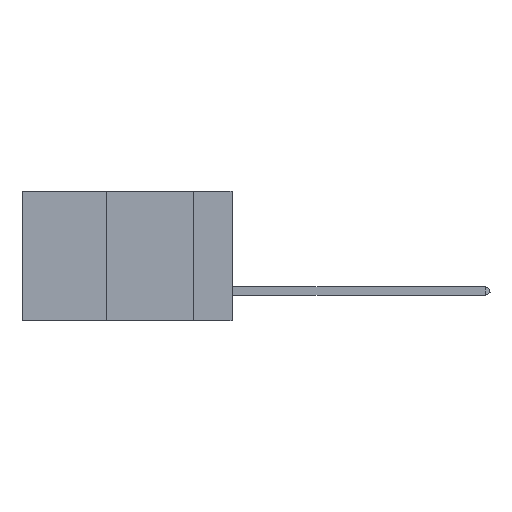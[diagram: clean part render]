
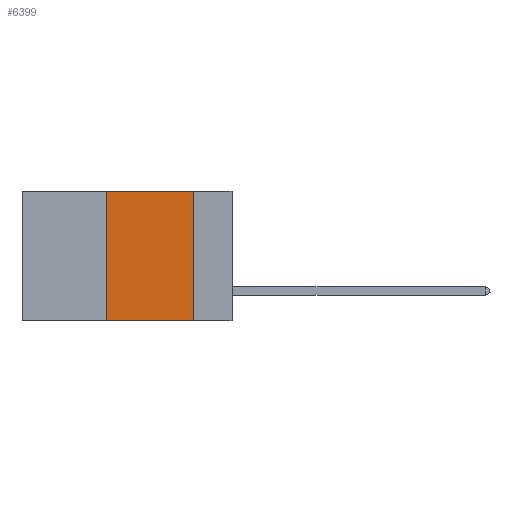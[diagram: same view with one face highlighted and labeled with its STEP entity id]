
A CAD part, left-side view. The second image highlights one B-rep face of the part: STEP entity #6399.
In plain terms, the highlighted planar face has unit normal (-1, 0, 0).
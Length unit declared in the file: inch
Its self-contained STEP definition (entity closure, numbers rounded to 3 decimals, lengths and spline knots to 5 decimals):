
#733 = ORIENTED_EDGE ( 'NONE', *, *, #5323, .T. ) ;
#735 = VECTOR ( 'NONE', #2194, 39.37008 ) ;
#1109 = ORIENTED_EDGE ( 'NONE', *, *, #1247, .F. ) ;
#1247 = EDGE_CURVE ( 'NONE', #1625, #7557, #7844, .T. ) ;
#1561 = LINE ( 'NONE', #7928, #9640 ) ;
#1625 = VERTEX_POINT ( 'NONE', #11867 ) ;
#1918 = VERTEX_POINT ( 'NONE', #10917 ) ;
#2194 = DIRECTION ( 'NONE',  ( 0., 0., -1. ) ) ;
#2244 = EDGE_CURVE ( 'NONE', #1918, #4324, #5093, .T. ) ;
#2353 = AXIS2_PLACEMENT_3D ( 'NONE', #8806, #9816, #11790 ) ;
#2877 = CARTESIAN_POINT ( 'NONE',  ( 0., 0.36, 0. ) ) ;
#3343 = VECTOR ( 'NONE', #7651, 39.37008 ) ;
#3532 = EDGE_LOOP ( 'NONE', ( #1109, #11764, #6362, #733 ) ) ;
#4320 = DIRECTION ( 'NONE',  ( 0., -1., 0. ) ) ;
#4324 = VERTEX_POINT ( 'NONE', #10662 ) ;
#5093 = LINE ( 'NONE', #2877, #10151 ) ;
#5323 = EDGE_CURVE ( 'NONE', #1918, #7557, #1561, .T. ) ;
#6362 = ORIENTED_EDGE ( 'NONE', *, *, #2244, .F. ) ;
#6399 = ADVANCED_FACE ( 'NONE', ( #8199 ), #7680, .F. ) ;
#7457 = LINE ( 'NONE', #10409, #3343 ) ;
#7557 = VERTEX_POINT ( 'NONE', #7798 ) ;
#7588 = DIRECTION ( 'NONE',  ( 0., 0., 1. ) ) ;
#7651 = DIRECTION ( 'NONE',  ( 0., -1., 0. ) ) ;
#7680 = PLANE ( 'NONE',  #2353 ) ;
#7798 = CARTESIAN_POINT ( 'NONE',  ( 0., 0.11, -0.37 ) ) ;
#7844 = LINE ( 'NONE', #7999, #735 ) ;
#7928 = CARTESIAN_POINT ( 'NONE',  ( 0., 0.6, -0.37 ) ) ;
#7999 = CARTESIAN_POINT ( 'NONE',  ( 0., 0.11, 0. ) ) ;
#8199 = FACE_OUTER_BOUND ( 'NONE', #3532, .T. ) ;
#8806 = CARTESIAN_POINT ( 'NONE',  ( 0., 0.6, 0. ) ) ;
#9640 = VECTOR ( 'NONE', #4320, 39.37008 ) ;
#9816 = DIRECTION ( 'NONE',  ( 1., 0., 0. ) ) ;
#10151 = VECTOR ( 'NONE', #7588, 39.37008 ) ;
#10409 = CARTESIAN_POINT ( 'NONE',  ( 0., 0.6, 0. ) ) ;
#10662 = CARTESIAN_POINT ( 'NONE',  ( 0., 0.36, 0. ) ) ;
#10917 = CARTESIAN_POINT ( 'NONE',  ( 0., 0.36, -0.37 ) ) ;
#11764 = ORIENTED_EDGE ( 'NONE', *, *, #11819, .F. ) ;
#11790 = DIRECTION ( 'NONE',  ( 0., 0., -1. ) ) ;
#11819 = EDGE_CURVE ( 'NONE', #4324, #1625, #7457, .T. ) ;
#11867 = CARTESIAN_POINT ( 'NONE',  ( 0., 0.11, 0. ) ) ;
